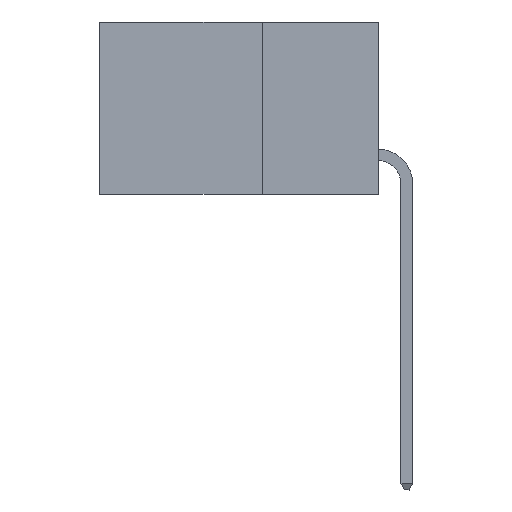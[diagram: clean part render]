
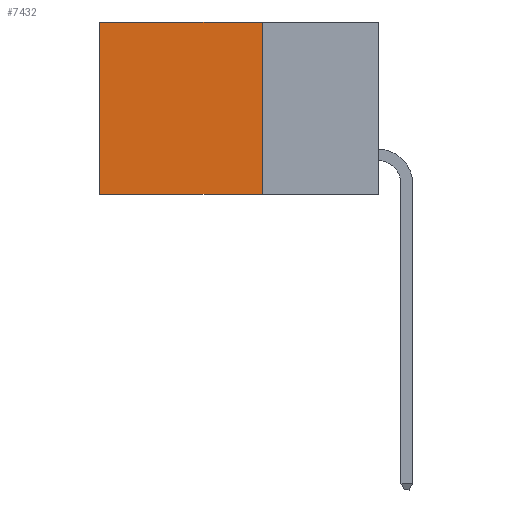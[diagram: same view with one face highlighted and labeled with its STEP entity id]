
A CAD part, left-side view. The second image highlights one B-rep face of the part: STEP entity #7432.
In plain terms, the highlighted planar face has unit normal (-1, 0, 0).
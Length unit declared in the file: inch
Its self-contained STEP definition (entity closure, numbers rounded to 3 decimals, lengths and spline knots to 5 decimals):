
#99 = VERTEX_POINT ( 'NONE', #6677 ) ;
#160 = CARTESIAN_POINT ( 'NONE',  ( 0.298, 0.6, -0.37 ) ) ;
#412 = LINE ( 'NONE', #5975, #9726 ) ;
#447 = DIRECTION ( 'NONE',  ( 0., 0., -1. ) ) ;
#614 = DIRECTION ( 'NONE',  ( 0., 1., 0. ) ) ;
#635 = CARTESIAN_POINT ( 'NONE',  ( 0.298, 0.25, 0. ) ) ;
#1145 = FACE_OUTER_BOUND ( 'NONE', #3185, .T. ) ;
#1185 = VECTOR ( 'NONE', #447, 39.37008 ) ;
#2587 = CARTESIAN_POINT ( 'NONE',  ( 0.298, 0.6, 0. ) ) ;
#2789 = VERTEX_POINT ( 'NONE', #4041 ) ;
#3043 = CARTESIAN_POINT ( 'NONE',  ( 0.298, 0.25, 0. ) ) ;
#3069 = EDGE_CURVE ( 'NONE', #2789, #6665, #9239, .T. ) ;
#3185 = EDGE_LOOP ( 'NONE', ( #4465, #6501, #8418, #8658 ) ) ;
#3370 = VECTOR ( 'NONE', #614, 39.37008 ) ;
#3792 = DIRECTION ( 'NONE',  ( 0., 0., -1. ) ) ;
#4041 = CARTESIAN_POINT ( 'NONE',  ( 0.298, 0.6, 0. ) ) ;
#4465 = ORIENTED_EDGE ( 'NONE', *, *, #3069, .T. ) ;
#4502 = AXIS2_PLACEMENT_3D ( 'NONE', #635, #8258, #3792 ) ;
#4985 = EDGE_CURVE ( 'NONE', #9553, #2789, #8296, .T. ) ;
#5033 = EDGE_CURVE ( 'NONE', #9553, #99, #412, .T. ) ;
#5243 = DIRECTION ( 'NONE',  ( 0., 1., 0. ) ) ;
#5282 = CARTESIAN_POINT ( 'NONE',  ( 0.298, 0.25, -0.37 ) ) ;
#5944 = DIRECTION ( 'NONE',  ( 0., 0., -1. ) ) ;
#5975 = CARTESIAN_POINT ( 'NONE',  ( 0.298, 0.25, 0. ) ) ;
#6066 = PLANE ( 'NONE',  #4502 ) ;
#6261 = CARTESIAN_POINT ( 'NONE',  ( 0.298, 0.25, 0. ) ) ;
#6383 = VECTOR ( 'NONE', #5243, 39.37008 ) ;
#6501 = ORIENTED_EDGE ( 'NONE', *, *, #8234, .F. ) ;
#6665 = VERTEX_POINT ( 'NONE', #160 ) ;
#6677 = CARTESIAN_POINT ( 'NONE',  ( 0.298, 0.25, -0.37 ) ) ;
#6913 = LINE ( 'NONE', #5282, #3370 ) ;
#7432 = ADVANCED_FACE ( 'NONE', ( #1145 ), #6066, .F. ) ;
#8234 = EDGE_CURVE ( 'NONE', #99, #6665, #6913, .T. ) ;
#8258 = DIRECTION ( 'NONE',  ( 1., 0., 0. ) ) ;
#8296 = LINE ( 'NONE', #6261, #6383 ) ;
#8418 = ORIENTED_EDGE ( 'NONE', *, *, #5033, .F. ) ;
#8658 = ORIENTED_EDGE ( 'NONE', *, *, #4985, .T. ) ;
#9239 = LINE ( 'NONE', #2587, #1185 ) ;
#9553 = VERTEX_POINT ( 'NONE', #3043 ) ;
#9726 = VECTOR ( 'NONE', #5944, 39.37008 ) ;
